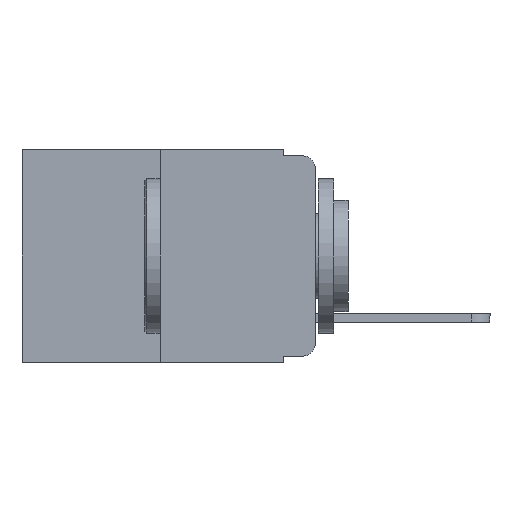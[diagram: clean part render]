
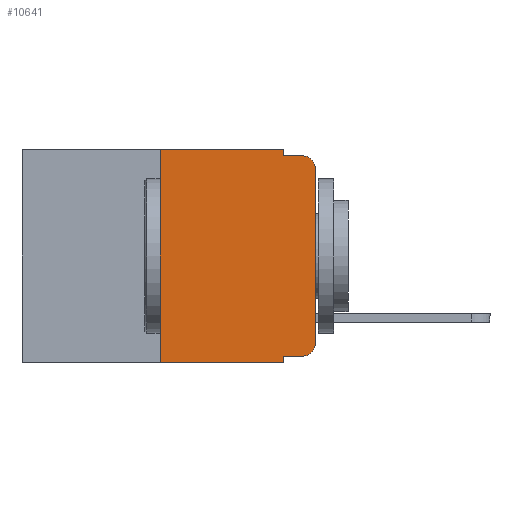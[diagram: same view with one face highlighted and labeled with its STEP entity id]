
A CAD part, left-side view. The second image highlights one B-rep face of the part: STEP entity #10641.
In plain terms, the highlighted planar face has unit normal (-1, 0, 0).
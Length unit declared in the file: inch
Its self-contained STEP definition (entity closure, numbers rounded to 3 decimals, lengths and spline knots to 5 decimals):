
#1 = CARTESIAN_POINT ( 'NONE',  ( 0., 0.051, 0. ) ) ;
#26 = LINE ( 'NONE', #168, #6553 ) ;
#152 = EDGE_CURVE ( 'NONE', #8776, #1468, #4956, .T. ) ;
#168 = CARTESIAN_POINT ( 'NONE',  ( 0., 0.051, 0. ) ) ;
#359 = DIRECTION ( 'NONE',  ( 0., 0., -1. ) ) ;
#1007 = EDGE_CURVE ( 'NONE', #8078, #8776, #12379, .T. ) ;
#1139 = ORIENTED_EDGE ( 'NONE', *, *, #11835, .T. ) ;
#1303 = VECTOR ( 'NONE', #11786, 39.37008 ) ;
#1468 = VERTEX_POINT ( 'NONE', #3163 ) ;
#1507 = EDGE_CURVE ( 'NONE', #11689, #14186, #1593, .T. ) ;
#1566 = VERTEX_POINT ( 'NONE', #14128 ) ;
#1593 = CIRCLE ( 'NONE', #2917, 0.02 ) ;
#1636 = VECTOR ( 'NONE', #7239, 39.37008 ) ;
#1714 = ORIENTED_EDGE ( 'NONE', *, *, #15506, .T. ) ;
#1873 = DIRECTION ( 'NONE',  ( 0., 0., -1. ) ) ;
#2022 = AXIS2_PLACEMENT_3D ( 'NONE', #10399, #3156, #11563 ) ;
#2110 = ORIENTED_EDGE ( 'NONE', *, *, #1507, .T. ) ;
#2300 = VECTOR ( 'NONE', #8226, 39.37008 ) ;
#2622 = LINE ( 'NONE', #2967, #14971 ) ;
#2688 = ORIENTED_EDGE ( 'NONE', *, *, #6744, .F. ) ;
#2793 = CARTESIAN_POINT ( 'NONE',  ( 0., 0.051, -0.01 ) ) ;
#2834 = VERTEX_POINT ( 'NONE', #14316 ) ;
#2917 = AXIS2_PLACEMENT_3D ( 'NONE', #5752, #14038, #6937 ) ;
#2967 = CARTESIAN_POINT ( 'NONE',  ( 0., 0.25, 0. ) ) ;
#3156 = DIRECTION ( 'NONE',  ( -1., 0., 0. ) ) ;
#3163 = CARTESIAN_POINT ( 'NONE',  ( 0., 0.02, -0.01 ) ) ;
#3185 = CARTESIAN_POINT ( 'NONE',  ( 0., 0.051, 0. ) ) ;
#3480 = ORIENTED_EDGE ( 'NONE', *, *, #11531, .F. ) ;
#3754 = FACE_OUTER_BOUND ( 'NONE', #10305, .T. ) ;
#4448 = ORIENTED_EDGE ( 'NONE', *, *, #152, .F. ) ;
#4942 = AXIS2_PLACEMENT_3D ( 'NONE', #15039, #9169, #1873 ) ;
#4956 = LINE ( 'NONE', #2793, #1636 ) ;
#4991 = LINE ( 'NONE', #6993, #1303 ) ;
#5013 = VERTEX_POINT ( 'NONE', #12765 ) ;
#5583 = LINE ( 'NONE', #11779, #2300 ) ;
#5752 = CARTESIAN_POINT ( 'NONE',  ( 0., 0.02, -0.313 ) ) ;
#5758 = EDGE_CURVE ( 'NONE', #2834, #8078, #4991, .T. ) ;
#5802 = CIRCLE ( 'NONE', #2022, 0.02 ) ;
#5965 = ORIENTED_EDGE ( 'NONE', *, *, #9800, .T. ) ;
#6553 = VECTOR ( 'NONE', #8715, 39.37008 ) ;
#6571 = CARTESIAN_POINT ( 'NONE',  ( 0., 0.02, -0.333 ) ) ;
#6744 = EDGE_CURVE ( 'NONE', #1566, #2834, #2622, .T. ) ;
#6937 = DIRECTION ( 'NONE',  ( 0., 0., -1. ) ) ;
#6971 = CARTESIAN_POINT ( 'NONE',  ( 0., 0., -0.313 ) ) ;
#6993 = CARTESIAN_POINT ( 'NONE',  ( 0., 0.473, 0. ) ) ;
#7134 = CARTESIAN_POINT ( 'NONE',  ( 0., 0.473, -0.343 ) ) ;
#7239 = DIRECTION ( 'NONE',  ( 0., -1., 0. ) ) ;
#7576 = VECTOR ( 'NONE', #14312, 39.37008 ) ;
#7933 = PLANE ( 'NONE',  #4942 ) ;
#8078 = VERTEX_POINT ( 'NONE', #1 ) ;
#8117 = VERTEX_POINT ( 'NONE', #9829 ) ;
#8226 = DIRECTION ( 'NONE',  ( 0., -1., 0. ) ) ;
#8379 = ORIENTED_EDGE ( 'NONE', *, *, #1007, .F. ) ;
#8658 = EDGE_CURVE ( 'NONE', #14186, #13744, #10763, .T. ) ;
#8715 = DIRECTION ( 'NONE',  ( 0., 0., -1. ) ) ;
#8754 = ORIENTED_EDGE ( 'NONE', *, *, #5758, .F. ) ;
#8776 = VERTEX_POINT ( 'NONE', #12253 ) ;
#9169 = DIRECTION ( 'NONE',  ( 1., 0., 0. ) ) ;
#9239 = VECTOR ( 'NONE', #359, 39.37008 ) ;
#9800 = EDGE_CURVE ( 'NONE', #1566, #5013, #10180, .T. ) ;
#9829 = CARTESIAN_POINT ( 'NONE',  ( 0., 0.051, -0.333 ) ) ;
#10180 = LINE ( 'NONE', #7134, #12935 ) ;
#10214 = DIRECTION ( 'NONE',  ( 0., 0., 1. ) ) ;
#10305 = EDGE_LOOP ( 'NONE', ( #13200, #1139, #4448, #8379, #8754, #2688, #5965, #3480, #1714, #2110 ) ) ;
#10399 = CARTESIAN_POINT ( 'NONE',  ( 0., 0.02, -0.03 ) ) ;
#10641 = ADVANCED_FACE ( 'NONE', ( #3754 ), #7933, .F. ) ;
#10763 = LINE ( 'NONE', #11950, #7576 ) ;
#11531 = EDGE_CURVE ( 'NONE', #8117, #5013, #26, .T. ) ;
#11563 = DIRECTION ( 'NONE',  ( 0., 0., -1. ) ) ;
#11689 = VERTEX_POINT ( 'NONE', #6571 ) ;
#11779 = CARTESIAN_POINT ( 'NONE',  ( 0., 0.051, -0.333 ) ) ;
#11786 = DIRECTION ( 'NONE',  ( 0., -1., 0. ) ) ;
#11835 = EDGE_CURVE ( 'NONE', #13744, #1468, #5802, .T. ) ;
#11914 = DIRECTION ( 'NONE',  ( 0., -1., 0. ) ) ;
#11950 = CARTESIAN_POINT ( 'NONE',  ( 0., 0., 0. ) ) ;
#12253 = CARTESIAN_POINT ( 'NONE',  ( 0., 0.051, -0.01 ) ) ;
#12379 = LINE ( 'NONE', #3185, #9239 ) ;
#12765 = CARTESIAN_POINT ( 'NONE',  ( 0., 0.051, -0.343 ) ) ;
#12935 = VECTOR ( 'NONE', #11914, 39.37008 ) ;
#13109 = CARTESIAN_POINT ( 'NONE',  ( 0., 0., -0.03 ) ) ;
#13200 = ORIENTED_EDGE ( 'NONE', *, *, #8658, .T. ) ;
#13744 = VERTEX_POINT ( 'NONE', #13109 ) ;
#14038 = DIRECTION ( 'NONE',  ( -1., 0., 0. ) ) ;
#14128 = CARTESIAN_POINT ( 'NONE',  ( 0., 0.25, -0.343 ) ) ;
#14186 = VERTEX_POINT ( 'NONE', #6971 ) ;
#14312 = DIRECTION ( 'NONE',  ( 0., 0., 1. ) ) ;
#14316 = CARTESIAN_POINT ( 'NONE',  ( 0., 0.25, 0. ) ) ;
#14971 = VECTOR ( 'NONE', #10214, 39.37008 ) ;
#15039 = CARTESIAN_POINT ( 'NONE',  ( 0., 0.473, 0. ) ) ;
#15506 = EDGE_CURVE ( 'NONE', #8117, #11689, #5583, .T. ) ;
